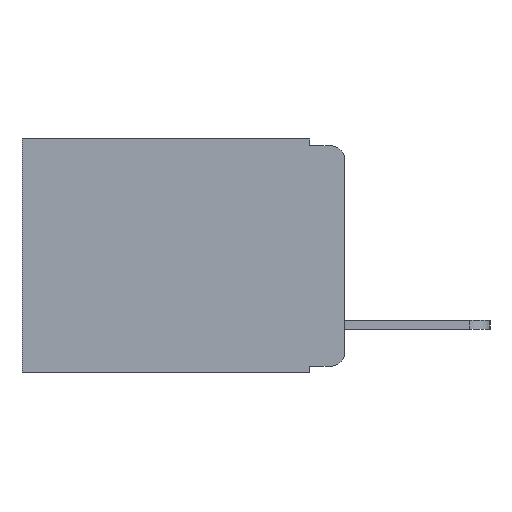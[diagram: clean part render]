
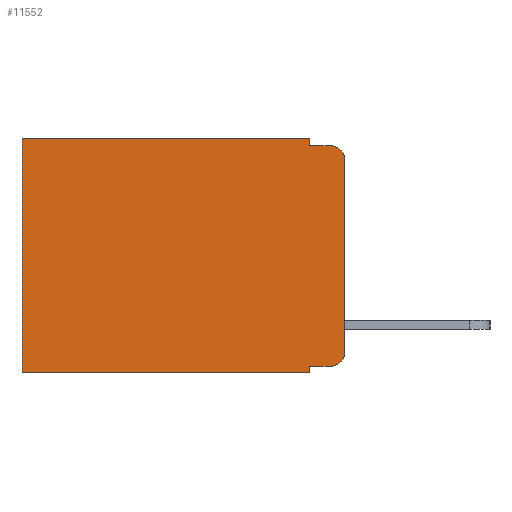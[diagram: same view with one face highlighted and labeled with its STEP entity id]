
A CAD part, left-side view. The second image highlights one B-rep face of the part: STEP entity #11552.
In plain terms, the highlighted planar face has unit normal (-1, 0, 0).
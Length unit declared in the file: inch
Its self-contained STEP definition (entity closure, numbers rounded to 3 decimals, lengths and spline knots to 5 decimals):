
#213 = EDGE_CURVE ( 'NONE', #1937, #3057, #11022, .T. ) ;
#233 = CARTESIAN_POINT ( 'NONE',  ( 0.298, 0.02, -0.333 ) ) ;
#357 = VERTEX_POINT ( 'NONE', #1674 ) ;
#615 = DIRECTION ( 'NONE',  ( 0., 1., 0. ) ) ;
#628 = CARTESIAN_POINT ( 'NONE',  ( 0.298, 0., -0.343 ) ) ;
#800 = PLANE ( 'NONE',  #9216 ) ;
#866 = VERTEX_POINT ( 'NONE', #7610 ) ;
#920 = ORIENTED_EDGE ( 'NONE', *, *, #213, .T. ) ;
#926 = ORIENTED_EDGE ( 'NONE', *, *, #1160, .T. ) ;
#1160 = EDGE_CURVE ( 'NONE', #9746, #2793, #9114, .T. ) ;
#1243 = VECTOR ( 'NONE', #2820, 39.37008 ) ;
#1639 = DIRECTION ( 'NONE',  ( -1., 0., 0. ) ) ;
#1674 = CARTESIAN_POINT ( 'NONE',  ( 0.298, 0.02, -0.01 ) ) ;
#1701 = CARTESIAN_POINT ( 'NONE',  ( 0.298, 0.051, 0. ) ) ;
#1714 = DIRECTION ( 'NONE',  ( 0., 0., -1. ) ) ;
#1720 = LINE ( 'NONE', #8424, #7054 ) ;
#1856 = VECTOR ( 'NONE', #3476, 39.37008 ) ;
#1937 = VERTEX_POINT ( 'NONE', #233 ) ;
#2039 = VERTEX_POINT ( 'NONE', #6318 ) ;
#2243 = LINE ( 'NONE', #1701, #9204 ) ;
#2347 = ORIENTED_EDGE ( 'NONE', *, *, #12018, .T. ) ;
#2617 = EDGE_CURVE ( 'NONE', #9746, #2039, #2243, .T. ) ;
#2643 = CARTESIAN_POINT ( 'NONE',  ( 0.298, 0.051, 0. ) ) ;
#2793 = VERTEX_POINT ( 'NONE', #10046 ) ;
#2820 = DIRECTION ( 'NONE',  ( 0., 1., 0. ) ) ;
#2926 = CARTESIAN_POINT ( 'NONE',  ( 0.298, 0.051, 0. ) ) ;
#3057 = VERTEX_POINT ( 'NONE', #11139 ) ;
#3318 = CARTESIAN_POINT ( 'NONE',  ( 0.298, 0.051, -0.333 ) ) ;
#3359 = FACE_OUTER_BOUND ( 'NONE', #7564, .T. ) ;
#3476 = DIRECTION ( 'NONE',  ( 0., -1., 0. ) ) ;
#4014 = DIRECTION ( 'NONE',  ( 0., 0., -1. ) ) ;
#4345 = CARTESIAN_POINT ( 'NONE',  ( 0.298, 0., -0.03 ) ) ;
#4415 = CARTESIAN_POINT ( 'NONE',  ( 0.298, 0.02, -0.03 ) ) ;
#4516 = EDGE_CURVE ( 'NONE', #2793, #10099, #4973, .T. ) ;
#4599 = DIRECTION ( 'NONE',  ( 0., 0., -1. ) ) ;
#4672 = ORIENTED_EDGE ( 'NONE', *, *, #2617, .F. ) ;
#4813 = EDGE_CURVE ( 'NONE', #866, #10099, #10058, .T. ) ;
#4930 = ORIENTED_EDGE ( 'NONE', *, *, #5635, .F. ) ;
#4952 = VECTOR ( 'NONE', #4599, 39.37008 ) ;
#4973 = LINE ( 'NONE', #10999, #9927 ) ;
#5064 = CARTESIAN_POINT ( 'NONE',  ( 0.298, 0.051, -0.01 ) ) ;
#5242 = DIRECTION ( 'NONE',  ( 0., -1., 0. ) ) ;
#5244 = LINE ( 'NONE', #2643, #4952 ) ;
#5393 = DIRECTION ( 'NONE',  ( 0., 0., -1. ) ) ;
#5396 = EDGE_CURVE ( 'NONE', #6772, #3057, #1720, .T. ) ;
#5635 = EDGE_CURVE ( 'NONE', #2039, #357, #6905, .T. ) ;
#5954 = EDGE_CURVE ( 'NONE', #10974, #866, #5244, .T. ) ;
#6209 = ORIENTED_EDGE ( 'NONE', *, *, #4813, .F. ) ;
#6318 = CARTESIAN_POINT ( 'NONE',  ( 0.298, 0.051, -0.01 ) ) ;
#6704 = LINE ( 'NONE', #3318, #10953 ) ;
#6772 = VERTEX_POINT ( 'NONE', #4345 ) ;
#6817 = CARTESIAN_POINT ( 'NONE',  ( 0.298, 0., 0. ) ) ;
#6905 = LINE ( 'NONE', #5064, #1856 ) ;
#7054 = VECTOR ( 'NONE', #7974, 39.37008 ) ;
#7188 = ORIENTED_EDGE ( 'NONE', *, *, #5954, .F. ) ;
#7196 = CARTESIAN_POINT ( 'NONE',  ( 0.298, 0.473, -0.343 ) ) ;
#7261 = EDGE_CURVE ( 'NONE', #10974, #1937, #6704, .T. ) ;
#7564 = EDGE_LOOP ( 'NONE', ( #11613, #2347, #4930, #4672, #926, #11111, #6209, #7188, #10306, #920 ) ) ;
#7593 = DIRECTION ( 'NONE',  ( 1., 0., 0. ) ) ;
#7610 = CARTESIAN_POINT ( 'NONE',  ( 0.298, 0.051, -0.343 ) ) ;
#7836 = AXIS2_PLACEMENT_3D ( 'NONE', #11531, #10760, #5393 ) ;
#7974 = DIRECTION ( 'NONE',  ( 0., 0., -1. ) ) ;
#8424 = CARTESIAN_POINT ( 'NONE',  ( 0.298, 0., 0. ) ) ;
#8977 = AXIS2_PLACEMENT_3D ( 'NONE', #4415, #1639, #1714 ) ;
#9114 = LINE ( 'NONE', #6817, #1243 ) ;
#9150 = CARTESIAN_POINT ( 'NONE',  ( 0.298, 0., 0. ) ) ;
#9204 = VECTOR ( 'NONE', #4014, 39.37008 ) ;
#9216 = AXIS2_PLACEMENT_3D ( 'NONE', #9150, #7593, #9501 ) ;
#9247 = VECTOR ( 'NONE', #615, 39.37008 ) ;
#9501 = DIRECTION ( 'NONE',  ( 0., 0., -1. ) ) ;
#9622 = CARTESIAN_POINT ( 'NONE',  ( 0.298, 0.051, -0.333 ) ) ;
#9746 = VERTEX_POINT ( 'NONE', #2926 ) ;
#9786 = DIRECTION ( 'NONE',  ( 0., 0., -1. ) ) ;
#9927 = VECTOR ( 'NONE', #9786, 39.37008 ) ;
#10046 = CARTESIAN_POINT ( 'NONE',  ( 0.298, 0.473, 0. ) ) ;
#10058 = LINE ( 'NONE', #628, #9247 ) ;
#10099 = VERTEX_POINT ( 'NONE', #7196 ) ;
#10306 = ORIENTED_EDGE ( 'NONE', *, *, #7261, .T. ) ;
#10760 = DIRECTION ( 'NONE',  ( -1., 0., 0. ) ) ;
#10838 = CIRCLE ( 'NONE', #8977, 0.02 ) ;
#10953 = VECTOR ( 'NONE', #5242, 39.37008 ) ;
#10974 = VERTEX_POINT ( 'NONE', #9622 ) ;
#10999 = CARTESIAN_POINT ( 'NONE',  ( 0.298, 0.473, 0. ) ) ;
#11022 = CIRCLE ( 'NONE', #7836, 0.02 ) ;
#11111 = ORIENTED_EDGE ( 'NONE', *, *, #4516, .T. ) ;
#11139 = CARTESIAN_POINT ( 'NONE',  ( 0.298, 0., -0.313 ) ) ;
#11531 = CARTESIAN_POINT ( 'NONE',  ( 0.298, 0.02, -0.313 ) ) ;
#11552 = ADVANCED_FACE ( 'NONE', ( #3359 ), #800, .F. ) ;
#11613 = ORIENTED_EDGE ( 'NONE', *, *, #5396, .F. ) ;
#12018 = EDGE_CURVE ( 'NONE', #6772, #357, #10838, .T. ) ;
